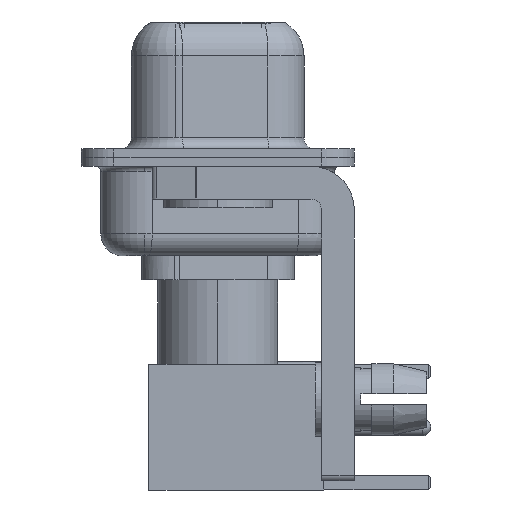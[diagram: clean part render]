
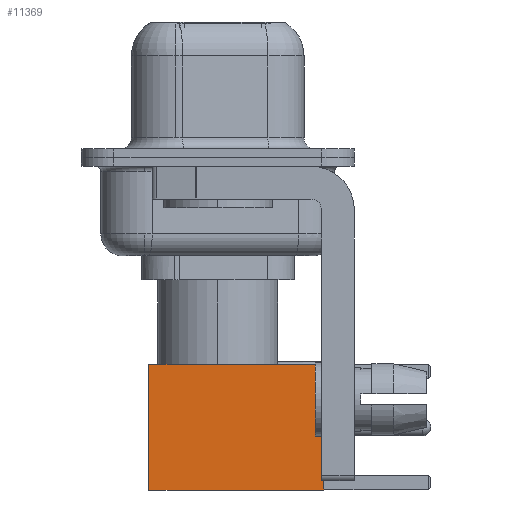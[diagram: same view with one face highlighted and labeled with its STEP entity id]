
A CAD part, left-side view. The second image highlights one B-rep face of the part: STEP entity #11369.
In plain terms, the highlighted face is planar.
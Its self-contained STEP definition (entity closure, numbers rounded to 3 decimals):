
#959 = FACE_OUTER_BOUND ( 'NONE', #12156, .T. ) ;
#1767 = VECTOR ( 'NONE', #9271, 1000. ) ;
#2272 = DIRECTION ( 'NONE',  ( -1., 0., 0. ) ) ;
#4125 = ORIENTED_EDGE ( 'NONE', *, *, #21283, .T. ) ;
#4988 = CARTESIAN_POINT ( 'NONE',  ( 2.875, 2.875, 0. ) ) ;
#5077 = ORIENTED_EDGE ( 'NONE', *, *, #18834, .F. ) ;
#5522 = AXIS2_PLACEMENT_3D ( 'NONE', #4988, #18635, #20228 ) ;
#6170 = ORIENTED_EDGE ( 'NONE', *, *, #14036, .F. ) ;
#6987 = LINE ( 'NONE', #22653, #11661 ) ;
#7587 = LINE ( 'NONE', #13452, #1767 ) ;
#9271 = DIRECTION ( 'NONE',  ( -1., 0., 0. ) ) ;
#9596 = EDGE_CURVE ( 'NONE', #10753, #27201, #6987, .T. ) ;
#10040 = CARTESIAN_POINT ( 'NONE',  ( -2.875, 2.875, 0. ) ) ;
#10682 = VERTEX_POINT ( 'NONE', #14568 ) ;
#10753 = VERTEX_POINT ( 'NONE', #25766 ) ;
#11369 = ADVANCED_FACE ( 'NONE', ( #959 ), #24664, .T. ) ;
#11661 = VECTOR ( 'NONE', #15902, 1000. ) ;
#12156 = EDGE_LOOP ( 'NONE', ( #28246, #4125, #6170, #5077 ) ) ;
#12163 = VECTOR ( 'NONE', #12214, 1000. ) ;
#12214 = DIRECTION ( 'NONE',  ( 0., 0., -1. ) ) ;
#12491 = LINE ( 'NONE', #10040, #12163 ) ;
#12569 = CARTESIAN_POINT ( 'NONE',  ( 2.875, 2.875, 0. ) ) ;
#13452 = CARTESIAN_POINT ( 'NONE',  ( 0., 2.875, 8. ) ) ;
#13490 = CARTESIAN_POINT ( 'NONE',  ( 0., 2.875, 0. ) ) ;
#14036 = EDGE_CURVE ( 'NONE', #21750, #10682, #12491, .T. ) ;
#14568 = CARTESIAN_POINT ( 'NONE',  ( -2.875, 2.875, 0. ) ) ;
#15902 = DIRECTION ( 'NONE',  ( 0., 0., -1. ) ) ;
#16771 = CARTESIAN_POINT ( 'NONE',  ( -2.875, 2.875, 8. ) ) ;
#17657 = LINE ( 'NONE', #13490, #18410 ) ;
#18410 = VECTOR ( 'NONE', #2272, 1000. ) ;
#18635 = DIRECTION ( 'NONE',  ( 0., 1., 0. ) ) ;
#18834 = EDGE_CURVE ( 'NONE', #10753, #21750, #7587, .T. ) ;
#20228 = DIRECTION ( 'NONE',  ( 0., 0., 1. ) ) ;
#21283 = EDGE_CURVE ( 'NONE', #27201, #10682, #17657, .T. ) ;
#21750 = VERTEX_POINT ( 'NONE', #16771 ) ;
#22653 = CARTESIAN_POINT ( 'NONE',  ( 2.875, 2.875, 0. ) ) ;
#24664 = PLANE ( 'NONE',  #5522 ) ;
#25766 = CARTESIAN_POINT ( 'NONE',  ( 2.875, 2.875, 8. ) ) ;
#27201 = VERTEX_POINT ( 'NONE', #12569 ) ;
#28246 = ORIENTED_EDGE ( 'NONE', *, *, #9596, .T. ) ;
